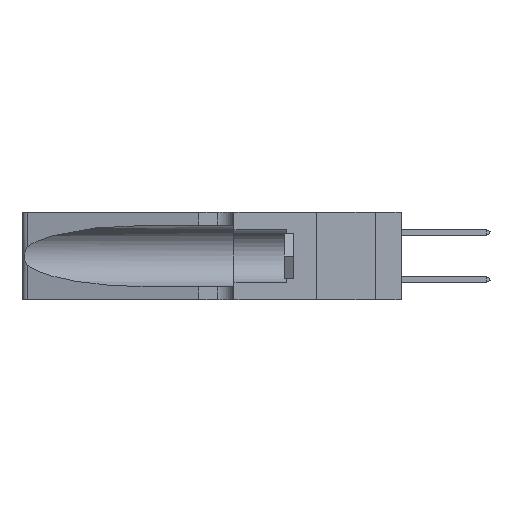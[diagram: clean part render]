
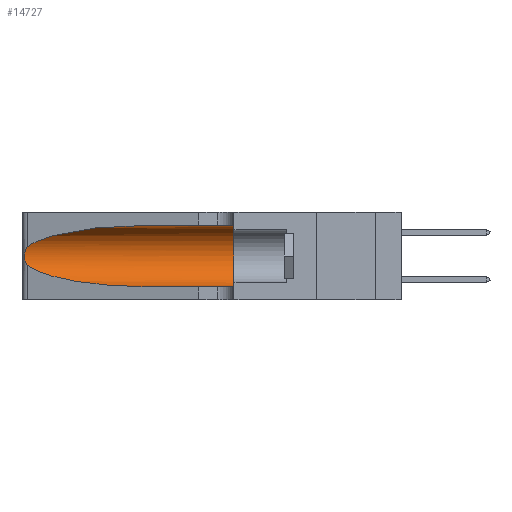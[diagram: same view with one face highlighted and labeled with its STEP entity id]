
A CAD part, left-side view. The second image highlights one B-rep face of the part: STEP entity #14727.
In plain terms, the highlighted cylindrical face has radius 3.308 mm (diameter 6.617 mm), a partial arc.
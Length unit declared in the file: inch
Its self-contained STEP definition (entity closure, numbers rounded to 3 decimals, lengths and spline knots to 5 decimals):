
#175 = CARTESIAN_POINT ( 'NONE',  ( 0.25555, 1.22993, 0.14849 ) ) ;
#475 = DIRECTION ( 'NONE',  ( 0., 1., 0. ) ) ;
#604 = ORIENTED_EDGE ( 'NONE', *, *, #12090, .F. ) ;
#2019 = LINE ( 'NONE', #23081, #23528 ) ;
#4823 = CARTESIAN_POINT ( 'NONE',  ( 0.25639, 1.23184, 0.21858 ) ) ;
#5408 = CARTESIAN_POINT ( 'NONE',  ( 0.18966, 0.96281, 0.31525 ) ) ;
#6673 = AXIS2_PLACEMENT_3D ( 'NONE', #15737, #20392, #24960 ) ;
#7174 = DIRECTION ( 'NONE',  ( 0., -1., 0. ) ) ;
#7316 = CARTESIAN_POINT ( 'NONE',  ( 0.26017, 1.23833, 0.17102 ) ) ;
#7368 = EDGE_CURVE ( 'NONE', #25425, #15413, #11683, .T. ) ;
#8621 = CIRCLE ( 'NONE', #14369, 0.13025 ) ;
#8995 = CARTESIAN_POINT ( 'NONE',  ( 0.25487, 1.22718, 0.14631 ) ) ;
#9265 = CARTESIAN_POINT ( 'NONE',  ( 0.26018, 1.23835, 0.19895 ) ) ;
#9500 = EDGE_CURVE ( 'NONE', #20680, #13184, #13405, .T. ) ;
#9670 = CARTESIAN_POINT ( 'NONE',  ( 0.25856, 1.23593, 0.16098 ) ) ;
#10412 = VECTOR ( 'NONE', #7174, 39.37008 ) ;
#10863 = ORIENTED_EDGE ( 'NONE', *, *, #15557, .T. ) ;
#11382 = CARTESIAN_POINT ( 'NONE',  ( 0.25487, 1.22718, 0.22369 ) ) ;
#11607 = FACE_OUTER_BOUND ( 'NONE', #28021, .T. ) ;
#11683 =( BOUNDED_CURVE ( )  B_SPLINE_CURVE ( 3, ( #12456, #5408, #14863, #26460 ),
 .UNSPECIFIED., .F., .F. ) 
 B_SPLINE_CURVE_WITH_KNOTS ( ( 4, 4 ),
 ( 1.5708, 2.84003 ),
 .UNSPECIFIED. ) 
 CURVE ( )  GEOMETRIC_REPRESENTATION_ITEM ( )  RATIONAL_B_SPLINE_CURVE ( ( 1., 0.87, 0.87, 1. ) ) 
 REPRESENTATION_ITEM ( '' )  );
#12090 = EDGE_CURVE ( 'NONE', #25425, #22479, #2019, .T. ) ;
#12358 = CARTESIAN_POINT ( 'NONE',  ( 0.1305, 1.61858, 0.05475 ) ) ;
#12456 = CARTESIAN_POINT ( 'NONE',  ( 0.1305, 0.72297, 0.31525 ) ) ;
#12939 = CARTESIAN_POINT ( 'NONE',  ( 0.2373, 1.15595, 0.08982 ) ) ;
#13184 = VERTEX_POINT ( 'NONE', #16404 ) ;
#13405 =( BOUNDED_CURVE ( )  B_SPLINE_CURVE ( 3, ( #22478, #12939, #27390, #17725 ),
 .UNSPECIFIED., .F., .F. ) 
 B_SPLINE_CURVE_WITH_KNOTS ( ( 4, 4 ),
 ( 3.44316, 4.71239 ),
 .UNSPECIFIED. ) 
 CURVE ( )  GEOMETRIC_REPRESENTATION_ITEM ( )  RATIONAL_B_SPLINE_CURVE ( ( 1., 0.87, 0.87, 1. ) ) 
 REPRESENTATION_ITEM ( '' )  );
#14091 = CARTESIAN_POINT ( 'NONE',  ( 0.25555, 1.22994, 0.2215 ) ) ;
#14283 = CARTESIAN_POINT ( 'NONE',  ( 0.25487, 1.22718, 0.14631 ) ) ;
#14369 = AXIS2_PLACEMENT_3D ( 'NONE', #15010, #475, #19860 ) ;
#14383 = CARTESIAN_POINT ( 'NONE',  ( 0.26075, 1.23896, 0.19203 ) ) ;
#14727 = ADVANCED_FACE ( 'NONE', ( #11607 ), #17569, .F. ) ;
#14863 = CARTESIAN_POINT ( 'NONE',  ( 0.2373, 1.15595, 0.28018 ) ) ;
#15010 = CARTESIAN_POINT ( 'NONE',  ( 0.1305, 0.35, 0.185 ) ) ;
#15149 = CARTESIAN_POINT ( 'NONE',  ( 0.1305, 0.35, 0.31525 ) ) ;
#15258 = ORIENTED_EDGE ( 'NONE', *, *, #28787, .T. ) ;
#15413 = VERTEX_POINT ( 'NONE', #11382 ) ;
#15557 = EDGE_CURVE ( 'NONE', #15413, #20680, #30531, .T. ) ;
#15737 = CARTESIAN_POINT ( 'NONE',  ( 0.1305, 1.61858, 0.185 ) ) ;
#16028 = ORIENTED_EDGE ( 'NONE', *, *, #7368, .T. ) ;
#16283 = VERTEX_POINT ( 'NONE', #29151 ) ;
#16404 = CARTESIAN_POINT ( 'NONE',  ( 0.1305, 0.72297, 0.05475 ) ) ;
#16892 = CARTESIAN_POINT ( 'NONE',  ( 0.25854, 1.2359, 0.20912 ) ) ;
#17569 = CYLINDRICAL_SURFACE ( 'NONE', #6673, 0.13025 ) ;
#17615 = CARTESIAN_POINT ( 'NONE',  ( 0.1305, 0.72297, 0.31525 ) ) ;
#17725 = CARTESIAN_POINT ( 'NONE',  ( 0.1305, 0.72297, 0.05475 ) ) ;
#18653 = ORIENTED_EDGE ( 'NONE', *, *, #28262, .F. ) ;
#18741 = CARTESIAN_POINT ( 'NONE',  ( 0.25789, 1.23486, 0.15765 ) ) ;
#18935 = CARTESIAN_POINT ( 'NONE',  ( 0.25487, 1.22718, 0.22369 ) ) ;
#19860 = DIRECTION ( 'NONE',  ( 0., 0., 1. ) ) ;
#20392 = DIRECTION ( 'NONE',  ( 0., -1., 0. ) ) ;
#20680 = VERTEX_POINT ( 'NONE', #8995 ) ;
#22478 = CARTESIAN_POINT ( 'NONE',  ( 0.25487, 1.22718, 0.14631 ) ) ;
#22479 = VERTEX_POINT ( 'NONE', #15149 ) ;
#23081 = CARTESIAN_POINT ( 'NONE',  ( 0.1305, 1.61858, 0.31525 ) ) ;
#23528 = VECTOR ( 'NONE', #27885, 39.37008 ) ;
#24960 = DIRECTION ( 'NONE',  ( 0., 0., -1. ) ) ;
#25425 = VERTEX_POINT ( 'NONE', #17615 ) ;
#26091 = CARTESIAN_POINT ( 'NONE',  ( 0.25639, 1.23186, 0.15144 ) ) ;
#26394 = LINE ( 'NONE', #12358, #10412 ) ;
#26460 = CARTESIAN_POINT ( 'NONE',  ( 0.25487, 1.22718, 0.22369 ) ) ;
#27390 = CARTESIAN_POINT ( 'NONE',  ( 0.18966, 0.96281, 0.05475 ) ) ;
#27885 = DIRECTION ( 'NONE',  ( 0., -1., 0. ) ) ;
#28021 = EDGE_LOOP ( 'NONE', ( #16028, #10863, #28391, #15258, #18653, #604 ) ) ;
#28262 = EDGE_CURVE ( 'NONE', #22479, #16283, #8621, .T. ) ;
#28391 = ORIENTED_EDGE ( 'NONE', *, *, #9500, .T. ) ;
#28598 = CARTESIAN_POINT ( 'NONE',  ( 0.25787, 1.23484, 0.2124 ) ) ;
#28700 = CARTESIAN_POINT ( 'NONE',  ( 0.26075, 1.23896, 0.178 ) ) ;
#28787 = EDGE_CURVE ( 'NONE', #13184, #16283, #26394, .T. ) ;
#29151 = CARTESIAN_POINT ( 'NONE',  ( 0.1305, 0.35, 0.05475 ) ) ;
#30531 = B_SPLINE_CURVE_WITH_KNOTS ( 'NONE', 3,
 ( #18935, #14091, #4823, #28598, #16892, #9265, #14383, #28700, #7316, #9670, #18741, #26091, #175, #14283 ),
 .UNSPECIFIED., .F., .F.,
 ( 4, 2, 2, 2, 2, 2, 4 ),
 ( 0., 0.00027, 0.00053, 0.00107, 0.0016, 0.00187, 0.00214 ),
 .UNSPECIFIED. ) ;
